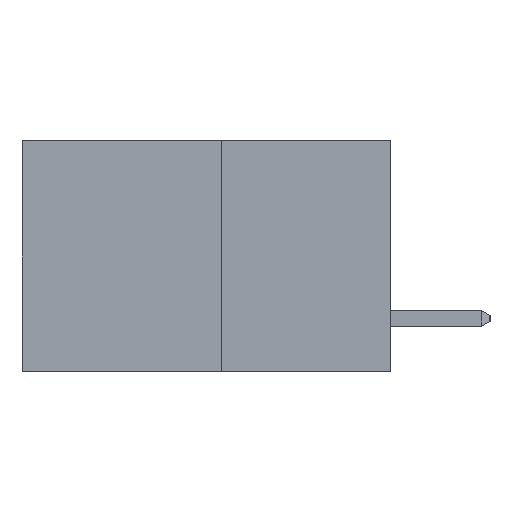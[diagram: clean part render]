
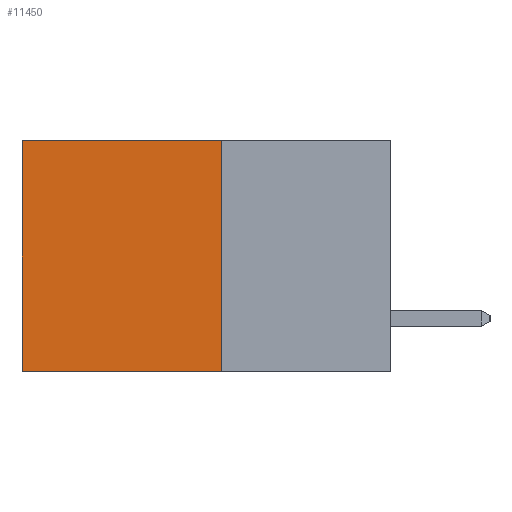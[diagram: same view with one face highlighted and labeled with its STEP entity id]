
A CAD part, left-side view. The second image highlights one B-rep face of the part: STEP entity #11450.
In plain terms, the highlighted planar face has unit normal (-1, 0, 0).
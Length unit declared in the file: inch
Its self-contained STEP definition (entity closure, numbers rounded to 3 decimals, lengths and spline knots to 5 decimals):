
#381 = VERTEX_POINT ( 'NONE', #6981 ) ;
#780 = LINE ( 'NONE', #10673, #10265 ) ;
#1042 = DIRECTION ( 'NONE',  ( 0., 0., -1. ) ) ;
#1056 = VECTOR ( 'NONE', #5247, 39.37008 ) ;
#2104 = PLANE ( 'NONE',  #5316 ) ;
#3276 = EDGE_CURVE ( 'NONE', #7764, #9414, #780, .T. ) ;
#3470 = DIRECTION ( 'NONE',  ( 0., 0., -1. ) ) ;
#3650 = CARTESIAN_POINT ( 'NONE',  ( 0.277, 0.59, -0.37 ) ) ;
#3709 = CARTESIAN_POINT ( 'NONE',  ( 0.277, 0.27, 0. ) ) ;
#3825 = LINE ( 'NONE', #9776, #1056 ) ;
#4155 = EDGE_CURVE ( 'NONE', #9414, #381, #11573, .T. ) ;
#4410 = LINE ( 'NONE', #9919, #11303 ) ;
#4986 = CARTESIAN_POINT ( 'NONE',  ( 0.277, 0.27, -0.37 ) ) ;
#5247 = DIRECTION ( 'NONE',  ( 0., 1., 0. ) ) ;
#5316 = AXIS2_PLACEMENT_3D ( 'NONE', #4986, #11258, #5928 ) ;
#5575 = ORIENTED_EDGE ( 'NONE', *, *, #9437, .F. ) ;
#5928 = DIRECTION ( 'NONE',  ( 0., 0., -1. ) ) ;
#6981 = CARTESIAN_POINT ( 'NONE',  ( 0.277, 0.59, -0.37 ) ) ;
#7147 = VERTEX_POINT ( 'NONE', #10074 ) ;
#7764 = VERTEX_POINT ( 'NONE', #3709 ) ;
#7913 = EDGE_LOOP ( 'NONE', ( #8799, #5575, #10694, #8816 ) ) ;
#8738 = VECTOR ( 'NONE', #1042, 39.37008 ) ;
#8799 = ORIENTED_EDGE ( 'NONE', *, *, #4155, .T. ) ;
#8816 = ORIENTED_EDGE ( 'NONE', *, *, #3276, .T. ) ;
#9121 = FACE_OUTER_BOUND ( 'NONE', #7913, .T. ) ;
#9414 = VERTEX_POINT ( 'NONE', #11449 ) ;
#9437 = EDGE_CURVE ( 'NONE', #7147, #381, #3825, .T. ) ;
#9758 = DIRECTION ( 'NONE',  ( 0., 1., 0. ) ) ;
#9776 = CARTESIAN_POINT ( 'NONE',  ( 0.277, 0.27, -0.37 ) ) ;
#9919 = CARTESIAN_POINT ( 'NONE',  ( 0.277, 0.27, -0.37 ) ) ;
#10060 = EDGE_CURVE ( 'NONE', #7764, #7147, #4410, .T. ) ;
#10074 = CARTESIAN_POINT ( 'NONE',  ( 0.277, 0.27, -0.37 ) ) ;
#10265 = VECTOR ( 'NONE', #9758, 39.37008 ) ;
#10673 = CARTESIAN_POINT ( 'NONE',  ( 0.277, 0.27, 0. ) ) ;
#10694 = ORIENTED_EDGE ( 'NONE', *, *, #10060, .F. ) ;
#11258 = DIRECTION ( 'NONE',  ( 1., 0., 0. ) ) ;
#11303 = VECTOR ( 'NONE', #3470, 39.37008 ) ;
#11449 = CARTESIAN_POINT ( 'NONE',  ( 0.277, 0.59, 0. ) ) ;
#11450 = ADVANCED_FACE ( 'NONE', ( #9121 ), #2104, .F. ) ;
#11573 = LINE ( 'NONE', #3650, #8738 ) ;
